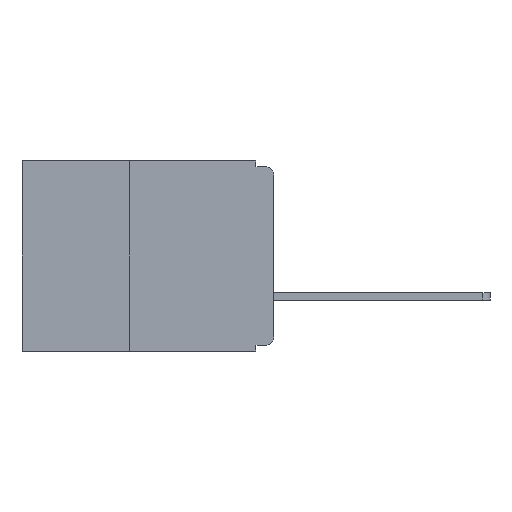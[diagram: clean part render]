
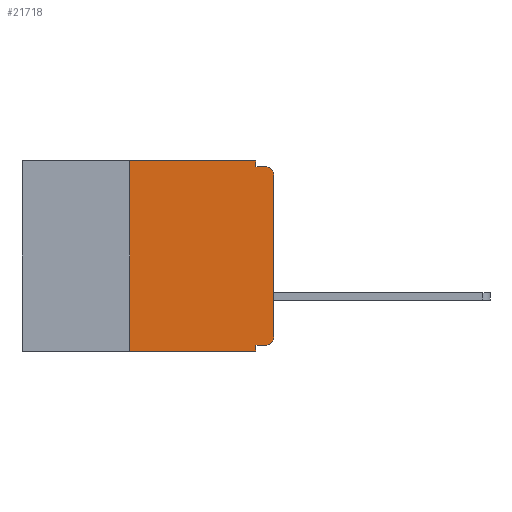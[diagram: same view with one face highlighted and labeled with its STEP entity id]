
A CAD part, left-side view. The second image highlights one B-rep face of the part: STEP entity #21718.
In plain terms, the highlighted planar face has unit normal (-1, 0, 0).
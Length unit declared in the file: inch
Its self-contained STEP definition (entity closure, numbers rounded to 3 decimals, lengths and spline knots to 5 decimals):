
#162 = CARTESIAN_POINT ( 'NONE',  ( 0., 0.031, -0.33 ) ) ;
#1026 = VERTEX_POINT ( 'NONE', #6585 ) ;
#1041 = EDGE_CURVE ( 'NONE', #22703, #13433, #16921, .T. ) ;
#1190 = CARTESIAN_POINT ( 'NONE',  ( 0., 0.031, 0. ) ) ;
#1724 = VERTEX_POINT ( 'NONE', #162 ) ;
#2089 = EDGE_CURVE ( 'NONE', #7067, #1026, #6170, .T. ) ;
#3693 = LINE ( 'NONE', #25029, #26612 ) ;
#3814 = DIRECTION ( 'NONE',  ( -1., 0., 0. ) ) ;
#3853 = DIRECTION ( 'NONE',  ( 0., 0., -1. ) ) ;
#4017 = VECTOR ( 'NONE', #5046, 39.37008 ) ;
#4241 = CARTESIAN_POINT ( 'NONE',  ( 0., 0., -0.025 ) ) ;
#4368 = VERTEX_POINT ( 'NONE', #20199 ) ;
#4582 = CARTESIAN_POINT ( 'NONE',  ( 0., 0.25, -0.33 ) ) ;
#4718 = CARTESIAN_POINT ( 'NONE',  ( 0., 0.437, -0.33 ) ) ;
#4756 = LINE ( 'NONE', #16761, #4017 ) ;
#4898 = CARTESIAN_POINT ( 'NONE',  ( 0., 0.25, 0. ) ) ;
#4947 = DIRECTION ( 'NONE',  ( 0., -1., 0. ) ) ;
#5046 = DIRECTION ( 'NONE',  ( 0., 0., 1. ) ) ;
#5066 = ORIENTED_EDGE ( 'NONE', *, *, #2089, .F. ) ;
#5415 = VECTOR ( 'NONE', #4947, 39.37008 ) ;
#5844 = EDGE_CURVE ( 'NONE', #14353, #1026, #15348, .T. ) ;
#5878 = DIRECTION ( 'NONE',  ( 0., 0., -1. ) ) ;
#6020 = VERTEX_POINT ( 'NONE', #4898 ) ;
#6170 = LINE ( 'NONE', #26174, #5415 ) ;
#6438 = ORIENTED_EDGE ( 'NONE', *, *, #9364, .F. ) ;
#6585 = CARTESIAN_POINT ( 'NONE',  ( 0., 0.015, -0.01 ) ) ;
#6613 = VECTOR ( 'NONE', #18830, 39.37008 ) ;
#7067 = VERTEX_POINT ( 'NONE', #29520 ) ;
#7712 = AXIS2_PLACEMENT_3D ( 'NONE', #15156, #3814, #3853 ) ;
#8128 = DIRECTION ( 'NONE',  ( 0., 0., -1. ) ) ;
#8161 = DIRECTION ( 'NONE',  ( -1., 0., 0. ) ) ;
#8166 = CARTESIAN_POINT ( 'NONE',  ( 0., 0.015, -0.025 ) ) ;
#8225 = EDGE_LOOP ( 'NONE', ( #10913, #29910, #5066, #25032, #16425, #21311, #22536, #6438, #29226, #14637 ) ) ;
#9282 = DIRECTION ( 'NONE',  ( 0., 0., 1. ) ) ;
#9364 = EDGE_CURVE ( 'NONE', #4368, #1724, #21116, .T. ) ;
#10328 = CARTESIAN_POINT ( 'NONE',  ( 0., 0.437, 0. ) ) ;
#10913 = ORIENTED_EDGE ( 'NONE', *, *, #21095, .T. ) ;
#10929 = EDGE_CURVE ( 'NONE', #22381, #1724, #25486, .T. ) ;
#13433 = VERTEX_POINT ( 'NONE', #28628 ) ;
#13715 = EDGE_CURVE ( 'NONE', #22703, #4368, #3693, .T. ) ;
#14119 = DIRECTION ( 'NONE',  ( 0., 0., -1. ) ) ;
#14353 = VERTEX_POINT ( 'NONE', #4241 ) ;
#14637 = ORIENTED_EDGE ( 'NONE', *, *, #1041, .T. ) ;
#15156 = CARTESIAN_POINT ( 'NONE',  ( 0., 0.015, -0.305 ) ) ;
#15348 = CIRCLE ( 'NONE', #20892, 0.015 ) ;
#15653 = EDGE_CURVE ( 'NONE', #22381, #6020, #26117, .T. ) ;
#16394 = PLANE ( 'NONE',  #18913 ) ;
#16425 = ORIENTED_EDGE ( 'NONE', *, *, #17226, .F. ) ;
#16761 = CARTESIAN_POINT ( 'NONE',  ( 0., 0., 0. ) ) ;
#16921 = CIRCLE ( 'NONE', #7712, 0.015 ) ;
#17226 = EDGE_CURVE ( 'NONE', #6020, #29232, #24576, .T. ) ;
#18830 = DIRECTION ( 'NONE',  ( 0., -1., 0. ) ) ;
#18867 = EDGE_CURVE ( 'NONE', #29232, #7067, #29249, .T. ) ;
#18913 = AXIS2_PLACEMENT_3D ( 'NONE', #21211, #28319, #14119 ) ;
#18999 = VECTOR ( 'NONE', #26892, 39.37008 ) ;
#19797 = VECTOR ( 'NONE', #9282, 39.37008 ) ;
#20199 = CARTESIAN_POINT ( 'NONE',  ( 0., 0.031, -0.32 ) ) ;
#20892 = AXIS2_PLACEMENT_3D ( 'NONE', #8166, #8161, #8128 ) ;
#21095 = EDGE_CURVE ( 'NONE', #13433, #14353, #4756, .T. ) ;
#21116 = LINE ( 'NONE', #22001, #26679 ) ;
#21211 = CARTESIAN_POINT ( 'NONE',  ( 0., 0.437, 0. ) ) ;
#21311 = ORIENTED_EDGE ( 'NONE', *, *, #15653, .F. ) ;
#21469 = CARTESIAN_POINT ( 'NONE',  ( 0., 0.25, -0.33 ) ) ;
#21718 = ADVANCED_FACE ( 'NONE', ( #29109 ), #16394, .F. ) ;
#22001 = CARTESIAN_POINT ( 'NONE',  ( 0., 0.031, -0.33 ) ) ;
#22381 = VERTEX_POINT ( 'NONE', #21469 ) ;
#22536 = ORIENTED_EDGE ( 'NONE', *, *, #10929, .T. ) ;
#22703 = VERTEX_POINT ( 'NONE', #25093 ) ;
#22996 = VECTOR ( 'NONE', #5878, 39.37008 ) ;
#24576 = LINE ( 'NONE', #10328, #18999 ) ;
#24908 = DIRECTION ( 'NONE',  ( 0., 0., -1. ) ) ;
#25029 = CARTESIAN_POINT ( 'NONE',  ( 0., 0., -0.32 ) ) ;
#25032 = ORIENTED_EDGE ( 'NONE', *, *, #18867, .F. ) ;
#25093 = CARTESIAN_POINT ( 'NONE',  ( 0., 0.015, -0.32 ) ) ;
#25486 = LINE ( 'NONE', #4718, #6613 ) ;
#26117 = LINE ( 'NONE', #4582, #19797 ) ;
#26174 = CARTESIAN_POINT ( 'NONE',  ( 0., 0., -0.01 ) ) ;
#26612 = VECTOR ( 'NONE', #29724, 39.37008 ) ;
#26679 = VECTOR ( 'NONE', #24908, 39.37008 ) ;
#26892 = DIRECTION ( 'NONE',  ( 0., -1., 0. ) ) ;
#28319 = DIRECTION ( 'NONE',  ( 1., 0., 0. ) ) ;
#28628 = CARTESIAN_POINT ( 'NONE',  ( 0., 0., -0.305 ) ) ;
#28817 = CARTESIAN_POINT ( 'NONE',  ( 0., 0.031, 0. ) ) ;
#29109 = FACE_OUTER_BOUND ( 'NONE', #8225, .T. ) ;
#29226 = ORIENTED_EDGE ( 'NONE', *, *, #13715, .F. ) ;
#29232 = VERTEX_POINT ( 'NONE', #28817 ) ;
#29249 = LINE ( 'NONE', #1190, #22996 ) ;
#29520 = CARTESIAN_POINT ( 'NONE',  ( 0., 0.031, -0.01 ) ) ;
#29724 = DIRECTION ( 'NONE',  ( 0., 1., 0. ) ) ;
#29910 = ORIENTED_EDGE ( 'NONE', *, *, #5844, .T. ) ;
